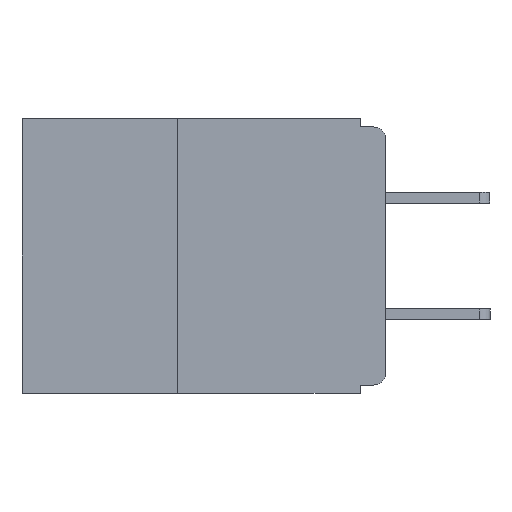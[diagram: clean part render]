
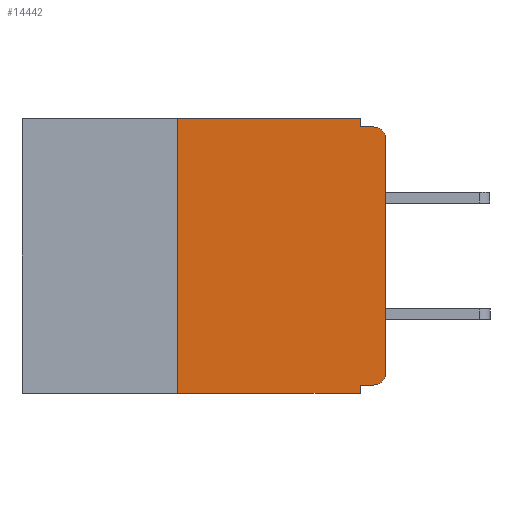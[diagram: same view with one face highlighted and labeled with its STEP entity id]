
A CAD part, left-side view. The second image highlights one B-rep face of the part: STEP entity #14442.
In plain terms, the highlighted planar face has unit normal (-1, 0, 0).
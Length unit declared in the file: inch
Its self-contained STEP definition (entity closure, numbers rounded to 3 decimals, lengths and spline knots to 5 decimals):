
#720 = ORIENTED_EDGE ( 'NONE', *, *, #4463, .F. ) ;
#886 = CARTESIAN_POINT ( 'NONE',  ( 0., 0.015, -0.025 ) ) ;
#1336 = VECTOR ( 'NONE', #10644, 39.37008 ) ;
#1787 = LINE ( 'NONE', #20835, #7545 ) ;
#2525 = ORIENTED_EDGE ( 'NONE', *, *, #14359, .F. ) ;
#2613 = VERTEX_POINT ( 'NONE', #17428 ) ;
#2712 = CARTESIAN_POINT ( 'NONE',  ( 0., 0., -0.305 ) ) ;
#2783 = ORIENTED_EDGE ( 'NONE', *, *, #24139, .T. ) ;
#3391 = DIRECTION ( 'NONE',  ( 0., 0., -1. ) ) ;
#3786 = CARTESIAN_POINT ( 'NONE',  ( 0., 0., 0. ) ) ;
#3928 = EDGE_CURVE ( 'NONE', #8562, #13331, #4707, .T. ) ;
#3932 = CARTESIAN_POINT ( 'NONE',  ( 0., 0.015, -0.32 ) ) ;
#4463 = EDGE_CURVE ( 'NONE', #22668, #8203, #21350, .T. ) ;
#4707 = CIRCLE ( 'NONE', #30409, 0.015 ) ;
#5045 = VERTEX_POINT ( 'NONE', #5428 ) ;
#5317 = ORIENTED_EDGE ( 'NONE', *, *, #15710, .F. ) ;
#5428 = CARTESIAN_POINT ( 'NONE',  ( 0., 0., -0.025 ) ) ;
#5510 = LINE ( 'NONE', #3786, #28197 ) ;
#6956 = PLANE ( 'NONE',  #26726 ) ;
#7002 = CIRCLE ( 'NONE', #14888, 0.015 ) ;
#7200 = DIRECTION ( 'NONE',  ( 0., 0., -1. ) ) ;
#7219 = ORIENTED_EDGE ( 'NONE', *, *, #10417, .T. ) ;
#7295 = DIRECTION ( 'NONE',  ( -1., 0., 0. ) ) ;
#7431 = CARTESIAN_POINT ( 'NONE',  ( 0., 0.015, -0.305 ) ) ;
#7545 = VECTOR ( 'NONE', #11518, 39.37008 ) ;
#7559 = CARTESIAN_POINT ( 'NONE',  ( 0., 0.25, -0.33 ) ) ;
#7653 = CARTESIAN_POINT ( 'NONE',  ( 0., 0.25, 0. ) ) ;
#7908 = VECTOR ( 'NONE', #19300, 39.37008 ) ;
#8203 = VERTEX_POINT ( 'NONE', #23837 ) ;
#8562 = VERTEX_POINT ( 'NONE', #3932 ) ;
#8620 = LINE ( 'NONE', #22422, #1336 ) ;
#9183 = EDGE_CURVE ( 'NONE', #13331, #5045, #5510, .T. ) ;
#9216 = ORIENTED_EDGE ( 'NONE', *, *, #21726, .F. ) ;
#9353 = DIRECTION ( 'NONE',  ( 0., -1., 0. ) ) ;
#9377 = DIRECTION ( 'NONE',  ( 1., 0., 0. ) ) ;
#10111 = EDGE_CURVE ( 'NONE', #8203, #23272, #15875, .T. ) ;
#10267 = ORIENTED_EDGE ( 'NONE', *, *, #3928, .T. ) ;
#10336 = ORIENTED_EDGE ( 'NONE', *, *, #10111, .F. ) ;
#10417 = EDGE_CURVE ( 'NONE', #22178, #2613, #26350, .T. ) ;
#10644 = DIRECTION ( 'NONE',  ( 0., 0., -1. ) ) ;
#11096 = DIRECTION ( 'NONE',  ( 0., 0., 1. ) ) ;
#11518 = DIRECTION ( 'NONE',  ( 0., 0., 1. ) ) ;
#13331 = VERTEX_POINT ( 'NONE', #2712 ) ;
#14054 = VECTOR ( 'NONE', #24867, 39.37008 ) ;
#14286 = LINE ( 'NONE', #23869, #7908 ) ;
#14359 = EDGE_CURVE ( 'NONE', #8562, #19542, #28075, .T. ) ;
#14368 = FACE_OUTER_BOUND ( 'NONE', #17075, .T. ) ;
#14437 = VECTOR ( 'NONE', #22295, 39.37008 ) ;
#14442 = ADVANCED_FACE ( 'NONE', ( #14368 ), #6956, .F. ) ;
#14888 = AXIS2_PLACEMENT_3D ( 'NONE', #886, #17723, #3391 ) ;
#15254 = ORIENTED_EDGE ( 'NONE', *, *, #9183, .T. ) ;
#15525 = EDGE_CURVE ( 'NONE', #22178, #28243, #1787, .T. ) ;
#15710 = EDGE_CURVE ( 'NONE', #28243, #22668, #14286, .T. ) ;
#15875 = LINE ( 'NONE', #27971, #22085 ) ;
#16098 = CARTESIAN_POINT ( 'NONE',  ( 0., 0., -0.32 ) ) ;
#16550 = VECTOR ( 'NONE', #20794, 39.37008 ) ;
#17075 = EDGE_LOOP ( 'NONE', ( #15254, #2783, #10336, #720, #5317, #20765, #7219, #9216, #2525, #10267 ) ) ;
#17428 = CARTESIAN_POINT ( 'NONE',  ( 0., 0.031, -0.33 ) ) ;
#17723 = DIRECTION ( 'NONE',  ( -1., 0., 0. ) ) ;
#19300 = DIRECTION ( 'NONE',  ( 0., -1., 0. ) ) ;
#19542 = VERTEX_POINT ( 'NONE', #25854 ) ;
#20765 = ORIENTED_EDGE ( 'NONE', *, *, #15525, .F. ) ;
#20794 = DIRECTION ( 'NONE',  ( 0., 1., 0. ) ) ;
#20835 = CARTESIAN_POINT ( 'NONE',  ( 0., 0.25, -0.33 ) ) ;
#21350 = LINE ( 'NONE', #28998, #14437 ) ;
#21726 = EDGE_CURVE ( 'NONE', #19542, #2613, #8620, .T. ) ;
#22085 = VECTOR ( 'NONE', #9353, 39.37008 ) ;
#22178 = VERTEX_POINT ( 'NONE', #7559 ) ;
#22295 = DIRECTION ( 'NONE',  ( 0., 0., -1. ) ) ;
#22422 = CARTESIAN_POINT ( 'NONE',  ( 0., 0.031, -0.33 ) ) ;
#22668 = VERTEX_POINT ( 'NONE', #23386 ) ;
#23272 = VERTEX_POINT ( 'NONE', #23346 ) ;
#23346 = CARTESIAN_POINT ( 'NONE',  ( 0., 0.015, -0.01 ) ) ;
#23386 = CARTESIAN_POINT ( 'NONE',  ( 0., 0.031, 0. ) ) ;
#23426 = CARTESIAN_POINT ( 'NONE',  ( 0., 0.437, 0. ) ) ;
#23837 = CARTESIAN_POINT ( 'NONE',  ( 0., 0.031, -0.01 ) ) ;
#23869 = CARTESIAN_POINT ( 'NONE',  ( 0., 0.437, 0. ) ) ;
#24139 = EDGE_CURVE ( 'NONE', #5045, #23272, #7002, .T. ) ;
#24867 = DIRECTION ( 'NONE',  ( 0., -1., 0. ) ) ;
#25707 = DIRECTION ( 'NONE',  ( 0., 0., -1. ) ) ;
#25854 = CARTESIAN_POINT ( 'NONE',  ( 0., 0.031, -0.32 ) ) ;
#26350 = LINE ( 'NONE', #29257, #14054 ) ;
#26726 = AXIS2_PLACEMENT_3D ( 'NONE', #23426, #9377, #25707 ) ;
#27971 = CARTESIAN_POINT ( 'NONE',  ( 0., 0., -0.01 ) ) ;
#28075 = LINE ( 'NONE', #16098, #16550 ) ;
#28197 = VECTOR ( 'NONE', #11096, 39.37008 ) ;
#28243 = VERTEX_POINT ( 'NONE', #7653 ) ;
#28998 = CARTESIAN_POINT ( 'NONE',  ( 0., 0.031, 0. ) ) ;
#29257 = CARTESIAN_POINT ( 'NONE',  ( 0., 0.437, -0.33 ) ) ;
#30409 = AXIS2_PLACEMENT_3D ( 'NONE', #7431, #7295, #7200 ) ;
